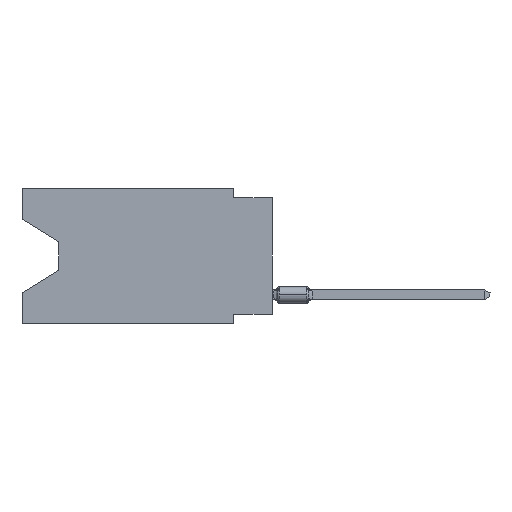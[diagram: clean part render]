
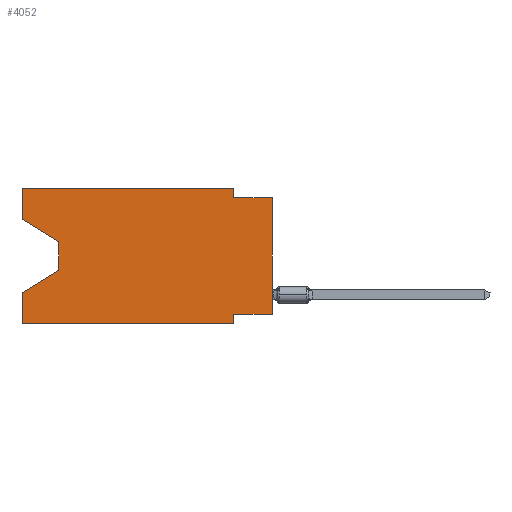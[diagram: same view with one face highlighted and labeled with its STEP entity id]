
A CAD part, left-side view. The second image highlights one B-rep face of the part: STEP entity #4052.
In plain terms, the highlighted planar face has unit normal (-1, 0, 0).
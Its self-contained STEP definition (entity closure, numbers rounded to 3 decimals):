
#928 = VERTEX_POINT ( 'NONE', #9427 ) ;
#2345 = ORIENTED_EDGE ( 'NONE', *, *, #4277, .T. ) ;
#2451 = VERTEX_POINT ( 'NONE', #15103 ) ;
#3280 = ORIENTED_EDGE ( 'NONE', *, *, #11608, .T. ) ;
#3850 = DIRECTION ( 'NONE',  ( 0., 0.855, -0.519 ) ) ;
#4052 = ADVANCED_FACE ( 'NONE', ( #16109 ), #10638, .F. ) ;
#4250 = CARTESIAN_POINT ( 'NONE',  ( 0., 16.383, -8.89 ) ) ;
#4277 = EDGE_CURVE ( 'NONE', #928, #25425, #26302, .T. ) ;
#4331 = LINE ( 'NONE', #13101, #14052 ) ;
#4380 = CARTESIAN_POINT ( 'NONE',  ( 0., 13.97, -5.385 ) ) ;
#4626 = CARTESIAN_POINT ( 'NONE',  ( 0., 0., -0.635 ) ) ;
#4801 = DIRECTION ( 'NONE',  ( 0., 0., -1. ) ) ;
#4844 = CARTESIAN_POINT ( 'NONE',  ( 0., 0., -0.635 ) ) ;
#4919 = LINE ( 'NONE', #18800, #19485 ) ;
#4938 = ORIENTED_EDGE ( 'NONE', *, *, #9565, .F. ) ;
#6729 = EDGE_CURVE ( 'NONE', #26326, #24793, #20108, .T. ) ;
#6892 = VECTOR ( 'NONE', #25950, 1000. ) ;
#7946 = CARTESIAN_POINT ( 'NONE',  ( 0., 2.54, -8.89 ) ) ;
#8659 = VECTOR ( 'NONE', #9995, 1000. ) ;
#8674 = CARTESIAN_POINT ( 'NONE',  ( 0., 0., -8.255 ) ) ;
#8900 = VECTOR ( 'NONE', #15705, 1000. ) ;
#9427 = CARTESIAN_POINT ( 'NONE',  ( 0., 16.383, -2.038 ) ) ;
#9565 = EDGE_CURVE ( 'NONE', #24948, #2451, #12706, .T. ) ;
#9809 = CARTESIAN_POINT ( 'NONE',  ( 0., 16.383, -8.89 ) ) ;
#9995 = DIRECTION ( 'NONE',  ( 0., -1., 0. ) ) ;
#10027 = VECTOR ( 'NONE', #15982, 1000. ) ;
#10229 = ORIENTED_EDGE ( 'NONE', *, *, #30229, .F. ) ;
#10348 = ORIENTED_EDGE ( 'NONE', *, *, #28214, .F. ) ;
#10359 = VECTOR ( 'NONE', #3850, 1000. ) ;
#10638 = PLANE ( 'NONE',  #23446 ) ;
#10811 = DIRECTION ( 'NONE',  ( 0., 0., -1. ) ) ;
#11608 = EDGE_CURVE ( 'NONE', #18711, #21433, #18381, .T. ) ;
#11631 = VERTEX_POINT ( 'NONE', #18022 ) ;
#12706 = LINE ( 'NONE', #21483, #27202 ) ;
#12978 = LINE ( 'NONE', #26655, #8900 ) ;
#13101 = CARTESIAN_POINT ( 'NONE',  ( 0., 16.383, 0. ) ) ;
#13128 = EDGE_CURVE ( 'NONE', #26326, #14250, #29368, .T. ) ;
#14052 = VECTOR ( 'NONE', #18216, 1000. ) ;
#14250 = VERTEX_POINT ( 'NONE', #4626 ) ;
#14932 = ORIENTED_EDGE ( 'NONE', *, *, #32016, .T. ) ;
#15103 = CARTESIAN_POINT ( 'NONE',  ( 0., 2.54, 0. ) ) ;
#15326 = DIRECTION ( 'NONE',  ( 0., 0., 1. ) ) ;
#15432 = ORIENTED_EDGE ( 'NONE', *, *, #31300, .F. ) ;
#15705 = DIRECTION ( 'NONE',  ( 0., 0., -1. ) ) ;
#15982 = DIRECTION ( 'NONE',  ( 0., -1., 0. ) ) ;
#16109 = FACE_OUTER_BOUND ( 'NONE', #21443, .T. ) ;
#16321 = ORIENTED_EDGE ( 'NONE', *, *, #32901, .F. ) ;
#16504 = CARTESIAN_POINT ( 'NONE',  ( 0., 13.97, -3.505 ) ) ;
#17124 = ORIENTED_EDGE ( 'NONE', *, *, #13128, .T. ) ;
#17193 = CARTESIAN_POINT ( 'NONE',  ( 0., 13.97, -5.385 ) ) ;
#18022 = CARTESIAN_POINT ( 'NONE',  ( 0., 16.383, -6.852 ) ) ;
#18216 = DIRECTION ( 'NONE',  ( 0., 0., 1. ) ) ;
#18381 = LINE ( 'NONE', #9809, #8659 ) ;
#18711 = VERTEX_POINT ( 'NONE', #4250 ) ;
#18800 = CARTESIAN_POINT ( 'NONE',  ( 0., 2.54, -8.89 ) ) ;
#19021 = ORIENTED_EDGE ( 'NONE', *, *, #35157, .F. ) ;
#19413 = VERTEX_POINT ( 'NONE', #23834 ) ;
#19485 = VECTOR ( 'NONE', #35007, 1000. ) ;
#19826 = VECTOR ( 'NONE', #32977, 1000. ) ;
#20108 = LINE ( 'NONE', #33760, #24493 ) ;
#20965 = CARTESIAN_POINT ( 'NONE',  ( 0., 16.383, 0. ) ) ;
#21433 = VERTEX_POINT ( 'NONE', #7946 ) ;
#21443 = EDGE_LOOP ( 'NONE', ( #2345, #35640, #14932, #15432, #3280, #19021, #31639, #17124, #16321, #10348, #4938, #10229 ) ) ;
#21483 = CARTESIAN_POINT ( 'NONE',  ( 0., 16.383, 0. ) ) ;
#23379 = DIRECTION ( 'NONE',  ( 0., 1., 0. ) ) ;
#23396 = VERTEX_POINT ( 'NONE', #17193 ) ;
#23446 = AXIS2_PLACEMENT_3D ( 'NONE', #27771, #30144, #10811 ) ;
#23834 = CARTESIAN_POINT ( 'NONE',  ( 0., 2.54, -0.635 ) ) ;
#24493 = VECTOR ( 'NONE', #23379, 1000. ) ;
#24793 = VERTEX_POINT ( 'NONE', #28670 ) ;
#24943 = VECTOR ( 'NONE', #4801, 1000. ) ;
#24948 = VERTEX_POINT ( 'NONE', #26105 ) ;
#25425 = VERTEX_POINT ( 'NONE', #16504 ) ;
#25727 = EDGE_CURVE ( 'NONE', #25425, #23396, #12978, .T. ) ;
#25950 = DIRECTION ( 'NONE',  ( 0., -0.855, -0.519 ) ) ;
#26105 = CARTESIAN_POINT ( 'NONE',  ( 0., 16.383, 0. ) ) ;
#26302 = LINE ( 'NONE', #29386, #6892 ) ;
#26326 = VERTEX_POINT ( 'NONE', #8674 ) ;
#26655 = CARTESIAN_POINT ( 'NONE',  ( 0., 13.97, -3.505 ) ) ;
#27202 = VECTOR ( 'NONE', #29671, 1000. ) ;
#27771 = CARTESIAN_POINT ( 'NONE',  ( 0., 16.383, 0. ) ) ;
#28214 = EDGE_CURVE ( 'NONE', #2451, #19413, #29797, .T. ) ;
#28670 = CARTESIAN_POINT ( 'NONE',  ( 0., 2.54, -8.255 ) ) ;
#29368 = LINE ( 'NONE', #34473, #32601 ) ;
#29386 = CARTESIAN_POINT ( 'NONE',  ( 0., 16.383, -2.038 ) ) ;
#29671 = DIRECTION ( 'NONE',  ( 0., -1., 0. ) ) ;
#29797 = LINE ( 'NONE', #35431, #24943 ) ;
#29899 = LINE ( 'NONE', #20965, #19826 ) ;
#30144 = DIRECTION ( 'NONE',  ( 1., 0., 0. ) ) ;
#30229 = EDGE_CURVE ( 'NONE', #928, #24948, #29899, .T. ) ;
#31300 = EDGE_CURVE ( 'NONE', #18711, #11631, #4331, .T. ) ;
#31639 = ORIENTED_EDGE ( 'NONE', *, *, #6729, .F. ) ;
#31930 = LINE ( 'NONE', #4380, #10359 ) ;
#32016 = EDGE_CURVE ( 'NONE', #23396, #11631, #31930, .T. ) ;
#32601 = VECTOR ( 'NONE', #15326, 1000. ) ;
#32901 = EDGE_CURVE ( 'NONE', #19413, #14250, #35478, .T. ) ;
#32977 = DIRECTION ( 'NONE',  ( 0., 0., 1. ) ) ;
#33760 = CARTESIAN_POINT ( 'NONE',  ( 0., 0., -8.255 ) ) ;
#34473 = CARTESIAN_POINT ( 'NONE',  ( 0., 0., 0. ) ) ;
#35007 = DIRECTION ( 'NONE',  ( 0., 0., -1. ) ) ;
#35157 = EDGE_CURVE ( 'NONE', #24793, #21433, #4919, .T. ) ;
#35431 = CARTESIAN_POINT ( 'NONE',  ( 0., 2.54, 0. ) ) ;
#35478 = LINE ( 'NONE', #4844, #10027 ) ;
#35640 = ORIENTED_EDGE ( 'NONE', *, *, #25727, .T. ) ;
